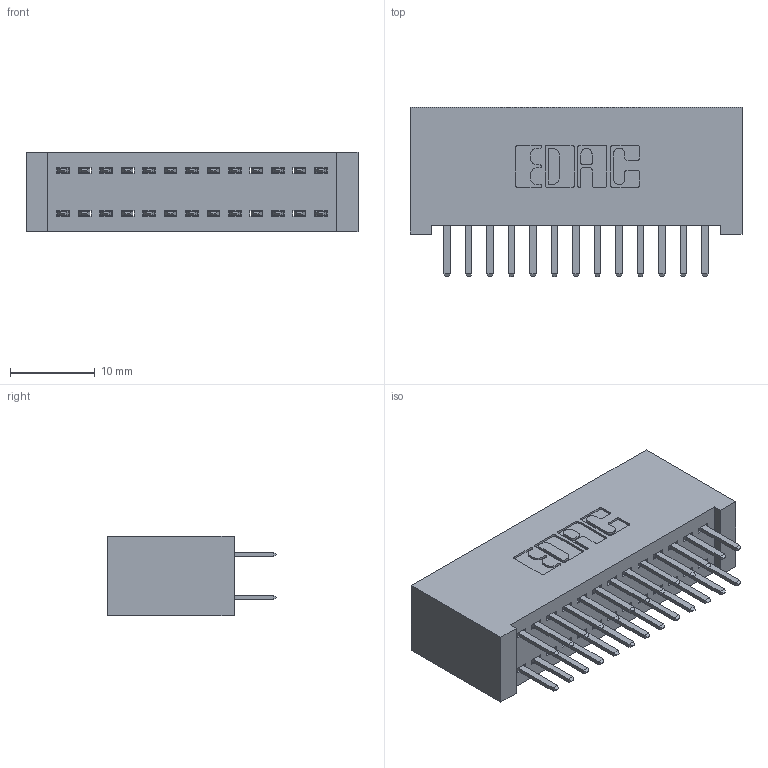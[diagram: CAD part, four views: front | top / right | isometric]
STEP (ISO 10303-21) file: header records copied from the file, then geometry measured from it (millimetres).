
FILE_DESCRIPTION (( 'STEP AP203' ), '1' );
FILE_NAME ('392-026-520-201.STEP', '2018-08-15T15:05:48', ( '' ), ( '' ), 'SwSTEP 2.0', 'SolidWorks 2016', '' );
FILE_SCHEMA (( 'CONFIG_CONTROL_DESIGN' ));
Length unit declared in the file: inch
Products named in the file (3): 345-292-001_345-293-120; 392-026-520-201; 342 Part_Lugless
Assembly tree (27 placements, depth 2):
  392-026-520-201
    342 Part_Lugless
    345-292-001_345-293-120  x26
Bounding box: 39.27 x 20.02 x 9.4 mm (x, y, z)
Volume: 3819.1 mm3; surface area: 5921.2 mm2
Topology: 27 solids, 27 shells, 1558 faces, 4513 edges, 2938 vertices
Faces by surface type: plane 1050, cylinder 508
Entity records: 11819 total; most frequent: CARTESIAN_POINT 2002, ORIENTED_EDGE 1926, DIRECTION 1743, EDGE_CURVE 963, VECTOR 839, LINE 839, VERTEX_POINT 638, AXIS2_PLACEMENT_3D 452
